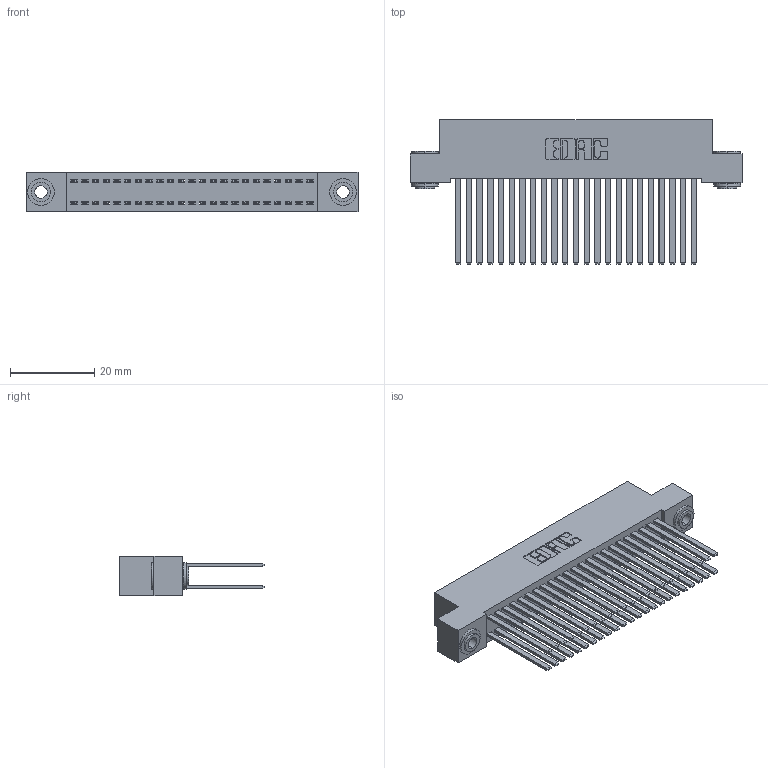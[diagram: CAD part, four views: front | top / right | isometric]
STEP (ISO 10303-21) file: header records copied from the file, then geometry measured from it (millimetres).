
FILE_DESCRIPTION (( 'STEP AP203' ), '1' );
FILE_NAME ('342-046-544-203.STEP', '2018-08-12T16:27:55', ( '' ), ( '' ), 'SwSTEP 2.0', 'SolidWorks 2016', '' );
FILE_SCHEMA (( 'CONFIG_CONTROL_DESIGN' ));
Length unit declared in the file: inch
Products named in the file (4): 345-292-001_345-293-144; 342-250-002_345-250-002-102; 342-046-544-203; 342 Part_.156 TH
Assembly tree (49 placements, depth 2):
  342-046-544-203
    342 Part_.156 TH
    345-292-001_345-293-144  x46
    342-250-002_345-250-002-102  x2
Bounding box: 78.74 x 34.3 x 9.4 mm (x, y, z)
Volume: 7652.5 mm3; surface area: 13988 mm2
Topology: 49 solids, 49 shells, 2264 faces, 6677 edges, 4386 vertices
Faces by surface type: plane 1548, cylinder 708, cone 8
Entity records: 17588 total; most frequent: CARTESIAN_POINT 2909, ORIENTED_EDGE 2838, DIRECTION 2549, EDGE_CURVE 1419, VECTOR 1271, LINE 1271, VERTEX_POINT 942, AXIS2_PLACEMENT_3D 639
